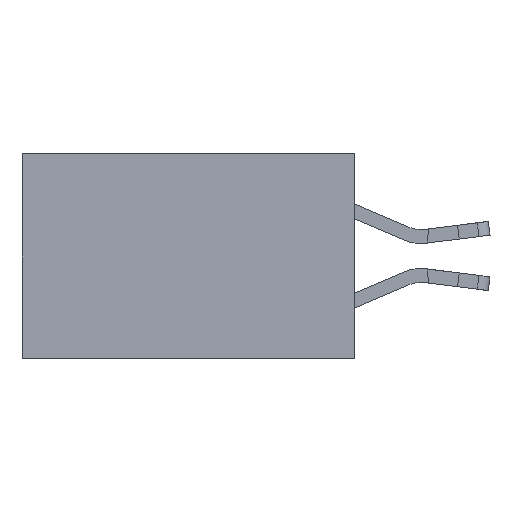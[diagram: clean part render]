
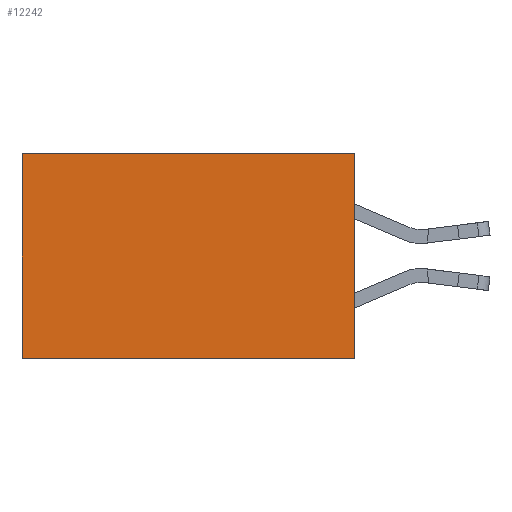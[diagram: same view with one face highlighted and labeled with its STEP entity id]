
A CAD part, left-side view. The second image highlights one B-rep face of the part: STEP entity #12242.
In plain terms, the highlighted planar face has unit normal (-1, 0, 0).
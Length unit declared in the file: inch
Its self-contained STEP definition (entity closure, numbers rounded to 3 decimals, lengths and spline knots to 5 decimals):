
#1597 = DIRECTION ( 'NONE',  ( 0., 0., -1. ) ) ;
#2603 = EDGE_CURVE ( 'NONE', #6556, #6896, #17242, .T. ) ;
#2894 = DIRECTION ( 'NONE',  ( 0., 0., -1. ) ) ;
#3828 = CARTESIAN_POINT ( 'NONE',  ( 0.2615, 0.6, -0.37 ) ) ;
#4315 = LINE ( 'NONE', #4404, #8999 ) ;
#4404 = CARTESIAN_POINT ( 'NONE',  ( 0.2615, 0.6, -0.37 ) ) ;
#6266 = EDGE_CURVE ( 'NONE', #9503, #6682, #17732, .T. ) ;
#6556 = VERTEX_POINT ( 'NONE', #10873 ) ;
#6682 = VERTEX_POINT ( 'NONE', #11968 ) ;
#6896 = VERTEX_POINT ( 'NONE', #3828 ) ;
#7177 = VECTOR ( 'NONE', #1597, 39.37008 ) ;
#7337 = LINE ( 'NONE', #8788, #7177 ) ;
#7414 = CARTESIAN_POINT ( 'NONE',  ( 0.2615, 0., 0. ) ) ;
#7656 = AXIS2_PLACEMENT_3D ( 'NONE', #9628, #9428, #15247 ) ;
#7719 = ORIENTED_EDGE ( 'NONE', *, *, #2603, .F. ) ;
#8771 = VECTOR ( 'NONE', #14596, 39.37008 ) ;
#8788 = CARTESIAN_POINT ( 'NONE',  ( 0.2615, 0., -0.37 ) ) ;
#8999 = VECTOR ( 'NONE', #2894, 39.37008 ) ;
#9428 = DIRECTION ( 'NONE',  ( 1., 0., 0. ) ) ;
#9503 = VERTEX_POINT ( 'NONE', #13703 ) ;
#9543 = ORIENTED_EDGE ( 'NONE', *, *, #14419, .F. ) ;
#9628 = CARTESIAN_POINT ( 'NONE',  ( 0.2615, 0., -0.37 ) ) ;
#10534 = ORIENTED_EDGE ( 'NONE', *, *, #6266, .T. ) ;
#10873 = CARTESIAN_POINT ( 'NONE',  ( 0.2615, 0., -0.37 ) ) ;
#10881 = ORIENTED_EDGE ( 'NONE', *, *, #13452, .T. ) ;
#11020 = VECTOR ( 'NONE', #13179, 39.37008 ) ;
#11136 = PLANE ( 'NONE',  #7656 ) ;
#11421 = CARTESIAN_POINT ( 'NONE',  ( 0.2615, 0., -0.37 ) ) ;
#11968 = CARTESIAN_POINT ( 'NONE',  ( 0.2615, 0.6, 0. ) ) ;
#12242 = ADVANCED_FACE ( 'NONE', ( #16299 ), #11136, .F. ) ;
#13179 = DIRECTION ( 'NONE',  ( 0., 1., 0. ) ) ;
#13452 = EDGE_CURVE ( 'NONE', #6682, #6896, #4315, .T. ) ;
#13703 = CARTESIAN_POINT ( 'NONE',  ( 0.2615, 0., 0. ) ) ;
#14419 = EDGE_CURVE ( 'NONE', #9503, #6556, #7337, .T. ) ;
#14596 = DIRECTION ( 'NONE',  ( 0., 1., 0. ) ) ;
#15247 = DIRECTION ( 'NONE',  ( 0., 0., -1. ) ) ;
#16299 = FACE_OUTER_BOUND ( 'NONE', #18132, .T. ) ;
#17242 = LINE ( 'NONE', #11421, #8771 ) ;
#17732 = LINE ( 'NONE', #7414, #11020 ) ;
#18132 = EDGE_LOOP ( 'NONE', ( #10881, #7719, #9543, #10534 ) ) ;
